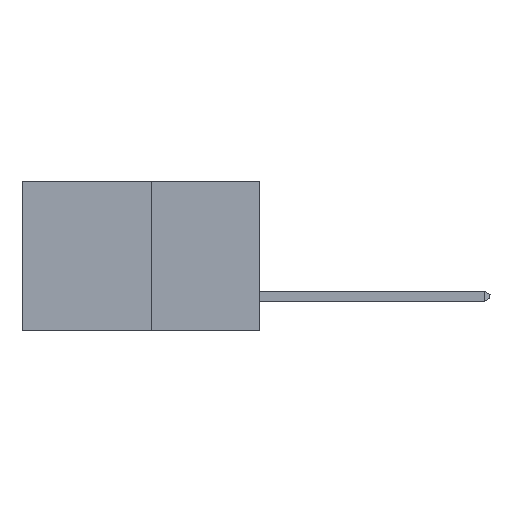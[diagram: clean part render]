
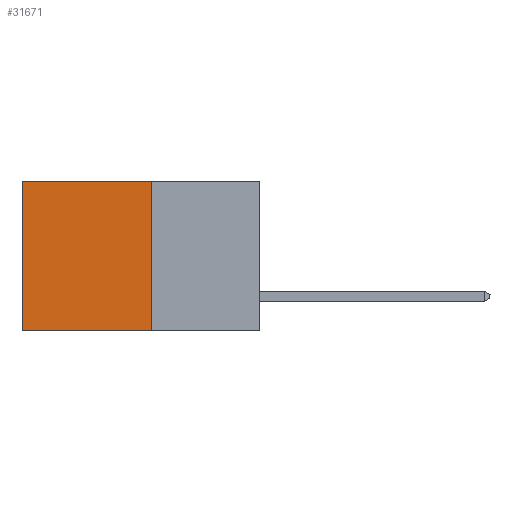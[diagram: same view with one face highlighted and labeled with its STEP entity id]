
A CAD part, left-side view. The second image highlights one B-rep face of the part: STEP entity #31671.
In plain terms, the highlighted planar face has unit normal (-1, 0, 0).
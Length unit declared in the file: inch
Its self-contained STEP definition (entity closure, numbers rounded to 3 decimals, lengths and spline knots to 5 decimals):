
#1395 = CARTESIAN_POINT ( 'NONE',  ( 0.277, 0.27, 0. ) ) ;
#1961 = DIRECTION ( 'NONE',  ( 0., 0., -1. ) ) ;
#2714 = EDGE_CURVE ( 'NONE', #18183, #12701, #3629, .T. ) ;
#3569 = ORIENTED_EDGE ( 'NONE', *, *, #2714, .T. ) ;
#3629 = LINE ( 'NONE', #23173, #29726 ) ;
#6008 = ORIENTED_EDGE ( 'NONE', *, *, #24869, .T. ) ;
#6614 = LINE ( 'NONE', #30189, #12564 ) ;
#6918 = CARTESIAN_POINT ( 'NONE',  ( 0.277, 0.27, -0.37 ) ) ;
#9472 = DIRECTION ( 'NONE',  ( 0., 0., -1. ) ) ;
#12098 = PLANE ( 'NONE',  #28319 ) ;
#12564 = VECTOR ( 'NONE', #12621, 39.37008 ) ;
#12621 = DIRECTION ( 'NONE',  ( 0., 1., 0. ) ) ;
#12701 = VERTEX_POINT ( 'NONE', #17646 ) ;
#13048 = LINE ( 'NONE', #6918, #25660 ) ;
#13936 = ORIENTED_EDGE ( 'NONE', *, *, #31024, .F. ) ;
#17239 = DIRECTION ( 'NONE',  ( 1., 0., 0. ) ) ;
#17646 = CARTESIAN_POINT ( 'NONE',  ( 0.277, 0.59, -0.37 ) ) ;
#18183 = VERTEX_POINT ( 'NONE', #24332 ) ;
#18377 = CARTESIAN_POINT ( 'NONE',  ( 0.277, 0.27, -0.37 ) ) ;
#18751 = DIRECTION ( 'NONE',  ( 0., 0., -1. ) ) ;
#18965 = DIRECTION ( 'NONE',  ( 0., 1., 0. ) ) ;
#20052 = VERTEX_POINT ( 'NONE', #1395 ) ;
#20545 = EDGE_LOOP ( 'NONE', ( #3569, #21836, #13936, #6008 ) ) ;
#20793 = VECTOR ( 'NONE', #18965, 39.37008 ) ;
#21836 = ORIENTED_EDGE ( 'NONE', *, *, #24541, .F. ) ;
#23173 = CARTESIAN_POINT ( 'NONE',  ( 0.277, 0.59, -0.37 ) ) ;
#23932 = CARTESIAN_POINT ( 'NONE',  ( 0.277, 0.27, 0. ) ) ;
#24332 = CARTESIAN_POINT ( 'NONE',  ( 0.277, 0.59, 0. ) ) ;
#24412 = FACE_OUTER_BOUND ( 'NONE', #20545, .T. ) ;
#24541 = EDGE_CURVE ( 'NONE', #31249, #12701, #6614, .T. ) ;
#24869 = EDGE_CURVE ( 'NONE', #20052, #18183, #27529, .T. ) ;
#25660 = VECTOR ( 'NONE', #9472, 39.37008 ) ;
#27529 = LINE ( 'NONE', #23932, #20793 ) ;
#28319 = AXIS2_PLACEMENT_3D ( 'NONE', #29785, #17239, #1961 ) ;
#29726 = VECTOR ( 'NONE', #18751, 39.37008 ) ;
#29785 = CARTESIAN_POINT ( 'NONE',  ( 0.277, 0.27, -0.37 ) ) ;
#30189 = CARTESIAN_POINT ( 'NONE',  ( 0.277, 0.27, -0.37 ) ) ;
#31024 = EDGE_CURVE ( 'NONE', #20052, #31249, #13048, .T. ) ;
#31249 = VERTEX_POINT ( 'NONE', #18377 ) ;
#31671 = ADVANCED_FACE ( 'NONE', ( #24412 ), #12098, .F. ) ;
